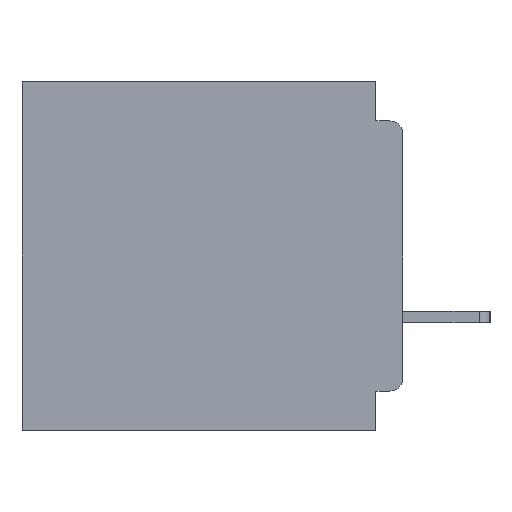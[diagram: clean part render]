
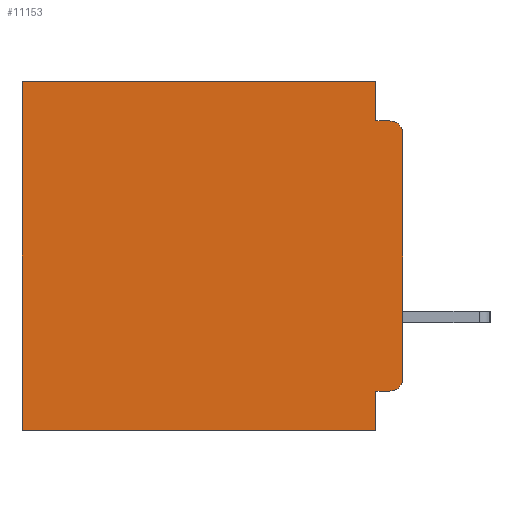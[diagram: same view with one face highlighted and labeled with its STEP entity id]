
A CAD part, left-side view. The second image highlights one B-rep face of the part: STEP entity #11153.
In plain terms, the highlighted planar face has unit normal (-1, 0, 0).
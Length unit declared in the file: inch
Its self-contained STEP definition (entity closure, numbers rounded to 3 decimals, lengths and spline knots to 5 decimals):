
#514 = DIRECTION ( 'NONE',  ( 0., -1., 0. ) ) ;
#682 = VERTEX_POINT ( 'NONE', #46811 ) ;
#1213 = ORIENTED_EDGE ( 'NONE', *, *, #47737, .T. ) ;
#1819 = CIRCLE ( 'NONE', #23625, 0.015 ) ;
#1828 = CARTESIAN_POINT ( 'NONE',  ( 0.3, 0., 0. ) ) ;
#2003 = DIRECTION ( 'NONE',  ( 0., 1., 0. ) ) ;
#3395 = DIRECTION ( 'NONE',  ( 1., 0., 0. ) ) ;
#3402 = LINE ( 'NONE', #25511, #27448 ) ;
#4071 = LINE ( 'NONE', #1828, #42176 ) ;
#6333 = ORIENTED_EDGE ( 'NONE', *, *, #14428, .F. ) ;
#7645 = VECTOR ( 'NONE', #2003, 39.37008 ) ;
#7822 = CARTESIAN_POINT ( 'NONE',  ( 0.3, 0.031, -0.4 ) ) ;
#8142 = CARTESIAN_POINT ( 'NONE',  ( 0.3, 0.031, 0. ) ) ;
#8771 = VECTOR ( 'NONE', #514, 39.37008 ) ;
#9522 = LINE ( 'NONE', #8142, #20784 ) ;
#10384 = EDGE_CURVE ( 'NONE', #23823, #28339, #3402, .T. ) ;
#11153 = ADVANCED_FACE ( 'NONE', ( #58418 ), #17721, .F. ) ;
#11767 = CARTESIAN_POINT ( 'NONE',  ( 0.3, 0., -0.4 ) ) ;
#13903 = CIRCLE ( 'NONE', #57896, 0.015 ) ;
#14232 = ORIENTED_EDGE ( 'NONE', *, *, #30134, .F. ) ;
#14428 = EDGE_CURVE ( 'NONE', #28339, #37283, #34695, .T. ) ;
#14517 = CARTESIAN_POINT ( 'NONE',  ( 0.3, 0.437, -0.4 ) ) ;
#14878 = CARTESIAN_POINT ( 'NONE',  ( 0.3, 0., -0.045 ) ) ;
#15779 = EDGE_CURVE ( 'NONE', #37283, #31746, #20400, .T. ) ;
#17721 = PLANE ( 'NONE',  #47576 ) ;
#18333 = CARTESIAN_POINT ( 'NONE',  ( 0.3, 0.015, -0.34 ) ) ;
#18595 = CARTESIAN_POINT ( 'NONE',  ( 0.3, 0.031, 0. ) ) ;
#18977 = CARTESIAN_POINT ( 'NONE',  ( 0.3, 0.015, -0.355 ) ) ;
#20308 = CARTESIAN_POINT ( 'NONE',  ( 0.3, 0., -0.06 ) ) ;
#20400 = LINE ( 'NONE', #11767, #7645 ) ;
#20733 = DIRECTION ( 'NONE',  ( 0., 1., 0. ) ) ;
#20784 = VECTOR ( 'NONE', #31966, 39.37008 ) ;
#20891 = CARTESIAN_POINT ( 'NONE',  ( 0.3, 0., -0.34 ) ) ;
#20951 = EDGE_CURVE ( 'NONE', #40966, #32394, #22206, .T. ) ;
#21532 = LINE ( 'NONE', #14878, #8771 ) ;
#22206 = LINE ( 'NONE', #33984, #46002 ) ;
#22305 = ORIENTED_EDGE ( 'NONE', *, *, #20951, .F. ) ;
#23120 = DIRECTION ( 'NONE',  ( 0., 0., -1. ) ) ;
#23625 = AXIS2_PLACEMENT_3D ( 'NONE', #57056, #28680, #61734 ) ;
#23823 = VERTEX_POINT ( 'NONE', #18977 ) ;
#25297 = VERTEX_POINT ( 'NONE', #52872 ) ;
#25511 = CARTESIAN_POINT ( 'NONE',  ( 0.3, 0., -0.355 ) ) ;
#27448 = VECTOR ( 'NONE', #20733, 39.37008 ) ;
#28339 = VERTEX_POINT ( 'NONE', #30748 ) ;
#28680 = DIRECTION ( 'NONE',  ( -1., 0., 0. ) ) ;
#29101 = DIRECTION ( 'NONE',  ( 0., 0., -1. ) ) ;
#29454 = ORIENTED_EDGE ( 'NONE', *, *, #35848, .T. ) ;
#30134 = EDGE_CURVE ( 'NONE', #57155, #30962, #9522, .T. ) ;
#30491 = VECTOR ( 'NONE', #29101, 39.37008 ) ;
#30574 = DIRECTION ( 'NONE',  ( 0., 1., 0. ) ) ;
#30748 = CARTESIAN_POINT ( 'NONE',  ( 0.3, 0.031, -0.355 ) ) ;
#30962 = VERTEX_POINT ( 'NONE', #38318 ) ;
#31376 = EDGE_LOOP ( 'NONE', ( #22305, #1213, #50662, #14232, #43973, #29454, #42835, #6333, #46639, #33391 ) ) ;
#31746 = VERTEX_POINT ( 'NONE', #44210 ) ;
#31966 = DIRECTION ( 'NONE',  ( 0., 0., -1. ) ) ;
#31995 = LINE ( 'NONE', #14517, #30491 ) ;
#32394 = VERTEX_POINT ( 'NONE', #20891 ) ;
#33391 = ORIENTED_EDGE ( 'NONE', *, *, #59997, .T. ) ;
#33984 = CARTESIAN_POINT ( 'NONE',  ( 0.3, 0., -0.4 ) ) ;
#34695 = LINE ( 'NONE', #55999, #58382 ) ;
#35848 = EDGE_CURVE ( 'NONE', #682, #31746, #31995, .T. ) ;
#36866 = DIRECTION ( 'NONE',  ( 0., 0., -1. ) ) ;
#37283 = VERTEX_POINT ( 'NONE', #7822 ) ;
#38318 = CARTESIAN_POINT ( 'NONE',  ( 0.3, 0.031, -0.045 ) ) ;
#38777 = DIRECTION ( 'NONE',  ( 0., 0., -1. ) ) ;
#40887 = EDGE_CURVE ( 'NONE', #30962, #25297, #21532, .T. ) ;
#40966 = VERTEX_POINT ( 'NONE', #20308 ) ;
#42176 = VECTOR ( 'NONE', #30574, 39.37008 ) ;
#42835 = ORIENTED_EDGE ( 'NONE', *, *, #15779, .F. ) ;
#43973 = ORIENTED_EDGE ( 'NONE', *, *, #54543, .T. ) ;
#44210 = CARTESIAN_POINT ( 'NONE',  ( 0.3, 0.437, -0.4 ) ) ;
#46002 = VECTOR ( 'NONE', #38777, 39.37008 ) ;
#46639 = ORIENTED_EDGE ( 'NONE', *, *, #10384, .F. ) ;
#46811 = CARTESIAN_POINT ( 'NONE',  ( 0.3, 0.437, 0. ) ) ;
#47576 = AXIS2_PLACEMENT_3D ( 'NONE', #50975, #3395, #36866 ) ;
#47737 = EDGE_CURVE ( 'NONE', #40966, #25297, #1819, .T. ) ;
#50662 = ORIENTED_EDGE ( 'NONE', *, *, #40887, .F. ) ;
#50975 = CARTESIAN_POINT ( 'NONE',  ( 0.3, 0., -0.4 ) ) ;
#51571 = DIRECTION ( 'NONE',  ( -1., 0., 0. ) ) ;
#52872 = CARTESIAN_POINT ( 'NONE',  ( 0.3, 0.015, -0.045 ) ) ;
#54543 = EDGE_CURVE ( 'NONE', #57155, #682, #4071, .T. ) ;
#55999 = CARTESIAN_POINT ( 'NONE',  ( 0.3, 0.031, -0.4 ) ) ;
#57056 = CARTESIAN_POINT ( 'NONE',  ( 0.3, 0.015, -0.06 ) ) ;
#57155 = VERTEX_POINT ( 'NONE', #18595 ) ;
#57896 = AXIS2_PLACEMENT_3D ( 'NONE', #18333, #51571, #23120 ) ;
#58382 = VECTOR ( 'NONE', #60703, 39.37008 ) ;
#58418 = FACE_OUTER_BOUND ( 'NONE', #31376, .T. ) ;
#59997 = EDGE_CURVE ( 'NONE', #23823, #32394, #13903, .T. ) ;
#60703 = DIRECTION ( 'NONE',  ( 0., 0., -1. ) ) ;
#61734 = DIRECTION ( 'NONE',  ( 0., 0., -1. ) ) ;
